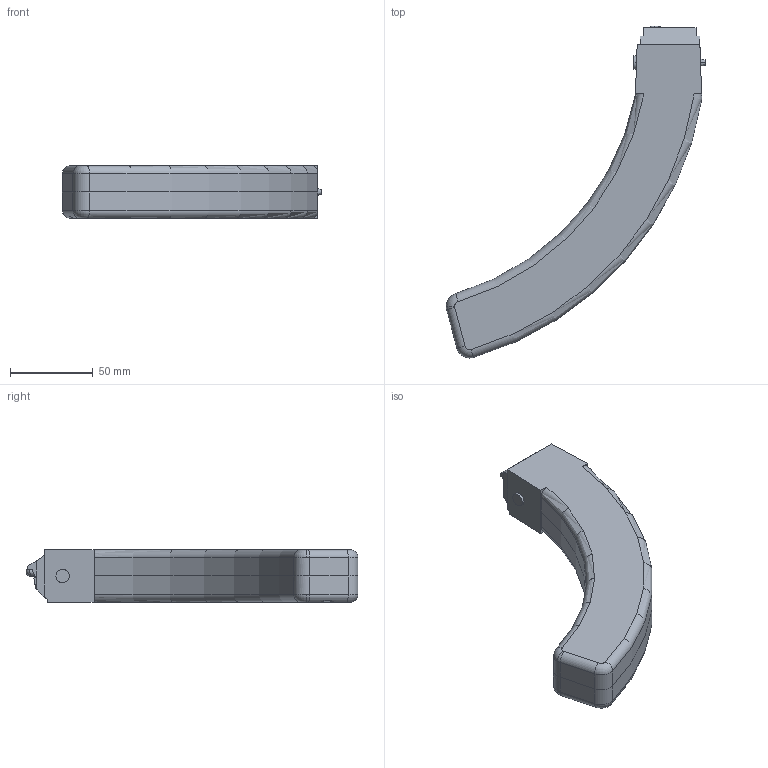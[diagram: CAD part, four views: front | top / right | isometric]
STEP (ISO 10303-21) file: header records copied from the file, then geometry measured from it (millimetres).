
FILE_DESCRIPTION (( 'STEP AP214' ), '1' );
FILE_NAME ('30rd_magazine.STEP', '2013-06-30T23:37:13', ( '' ), ( '' ), 'SwSTEP 2.0', 'SolidWorks 2013', '' );
FILE_SCHEMA (( 'AUTOMOTIVE_DESIGN' ));
Length unit declared in the file: millimetre
Products named in the file (8): 22LR; 22LR-Bullet; 22LR-Case; roller; follower; left; right; 30rd_magazine
Assembly tree (7 placements, depth 3):
  30rd_magazine
    right
    left
    follower
    roller
    22LR
      22LR-Case
      22LR-Bullet
Bounding box: 156.86 x 200.65 x 32 mm (x, y, z)
Volume: 164535.3 mm3; surface area: 96183.5 mm2
Topology: 6 solids, 6 shells, 342 faces, 925 edges, 596 vertices
Faces by surface type: plane 196, cylinder 112, torus 25, sphere 4, bspline 3, cone 2
Entity records: 11264 total; most frequent: CARTESIAN_POINT 2212, DIRECTION 1885, ORIENTED_EDGE 1838, EDGE_CURVE 919, AXIS2_PLACEMENT_3D 658, VERTEX_POINT 596, VECTOR 569, LINE 569
